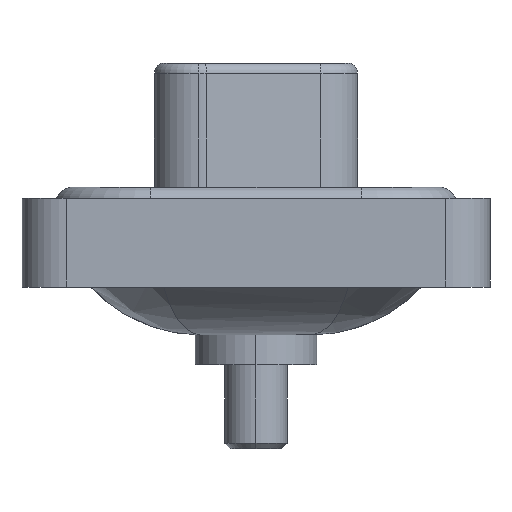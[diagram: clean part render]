
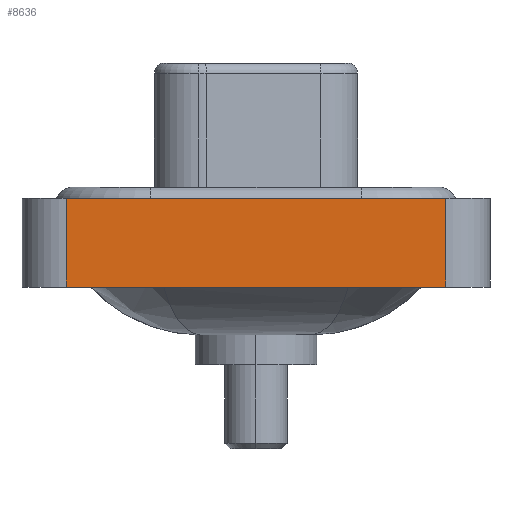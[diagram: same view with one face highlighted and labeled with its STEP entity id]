
A CAD part, left-side view. The second image highlights one B-rep face of the part: STEP entity #8636.
In plain terms, the highlighted planar face has unit normal (-1, 0, 0).
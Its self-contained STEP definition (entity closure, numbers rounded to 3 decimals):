
#46 = CARTESIAN_POINT ( 'NONE',  ( -7.25, -8.55, -3.6 ) ) ;
#83 = EDGE_CURVE ( 'NONE', #11036, #11144, #6718, .T. ) ;
#249 = CARTESIAN_POINT ( 'NONE',  ( -7.25, -8.55, -3.6 ) ) ;
#253 = EDGE_CURVE ( 'NONE', #9072, #11144, #12632, .T. ) ;
#1643 = CARTESIAN_POINT ( 'NONE',  ( -7.25, 8.55, -3.6 ) ) ;
#2103 = VECTOR ( 'NONE', #5827, 1000. ) ;
#2642 = DIRECTION ( 'NONE',  ( 0., -1., 0. ) ) ;
#3257 = CARTESIAN_POINT ( 'NONE',  ( -7.25, -8.55, 0.4 ) ) ;
#4572 = VECTOR ( 'NONE', #4865, 1000. ) ;
#4865 = DIRECTION ( 'NONE',  ( 0., 0., 1. ) ) ;
#4921 = ORIENTED_EDGE ( 'NONE', *, *, #8899, .T. ) ;
#5324 = VECTOR ( 'NONE', #2642, 1000. ) ;
#5597 = CARTESIAN_POINT ( 'NONE',  ( -7.25, 8.55, 0.4 ) ) ;
#5620 = EDGE_CURVE ( 'NONE', #14416, #11036, #13034, .T. ) ;
#5827 = DIRECTION ( 'NONE',  ( 0., 0., 1. ) ) ;
#6493 = DIRECTION ( 'NONE',  ( 0., -1., 0. ) ) ;
#6599 = EDGE_LOOP ( 'NONE', ( #6995, #10084, #9593, #4921 ) ) ;
#6718 = LINE ( 'NONE', #7648, #7007 ) ;
#6995 = ORIENTED_EDGE ( 'NONE', *, *, #253, .T. ) ;
#7007 = VECTOR ( 'NONE', #6493, 1000. ) ;
#7057 = DIRECTION ( 'NONE',  ( -1., 0., 0. ) ) ;
#7648 = CARTESIAN_POINT ( 'NONE',  ( -7.25, -8.55, 0.4 ) ) ;
#8636 = ADVANCED_FACE ( 'NONE', ( #12743 ), #11688, .T. ) ;
#8899 = EDGE_CURVE ( 'NONE', #14416, #9072, #11844, .T. ) ;
#9072 = VERTEX_POINT ( 'NONE', #46 ) ;
#9492 = CARTESIAN_POINT ( 'NONE',  ( -7.25, -8.55, -3.6 ) ) ;
#9593 = ORIENTED_EDGE ( 'NONE', *, *, #5620, .F. ) ;
#10084 = ORIENTED_EDGE ( 'NONE', *, *, #83, .F. ) ;
#11036 = VERTEX_POINT ( 'NONE', #5597 ) ;
#11144 = VERTEX_POINT ( 'NONE', #3257 ) ;
#11688 = PLANE ( 'NONE',  #12580 ) ;
#11844 = LINE ( 'NONE', #13040, #5324 ) ;
#12580 = AXIS2_PLACEMENT_3D ( 'NONE', #9492, #7057, #14105 ) ;
#12632 = LINE ( 'NONE', #249, #4572 ) ;
#12743 = FACE_OUTER_BOUND ( 'NONE', #6599, .T. ) ;
#13034 = LINE ( 'NONE', #14100, #2103 ) ;
#13040 = CARTESIAN_POINT ( 'NONE',  ( -7.25, -8.55, -3.6 ) ) ;
#14100 = CARTESIAN_POINT ( 'NONE',  ( -7.25, 8.55, -3.6 ) ) ;
#14105 = DIRECTION ( 'NONE',  ( 0., 0., 1. ) ) ;
#14416 = VERTEX_POINT ( 'NONE', #1643 ) ;
